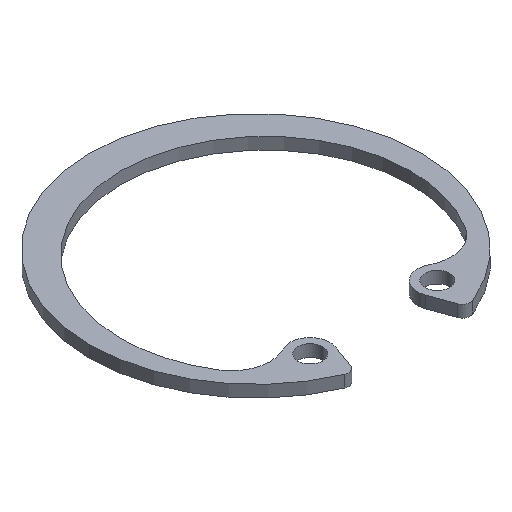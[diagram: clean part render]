
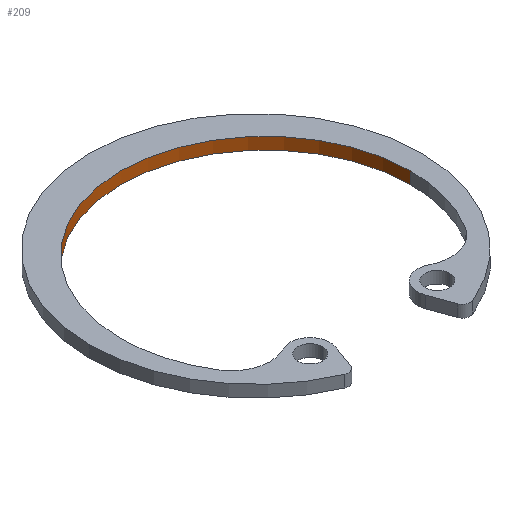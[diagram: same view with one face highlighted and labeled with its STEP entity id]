
A CAD part, isometric view. The second image highlights one B-rep face of the part: STEP entity #209.
In plain terms, the highlighted cylindrical face has radius 14.6 mm (diameter 29.199 mm), a partial arc.
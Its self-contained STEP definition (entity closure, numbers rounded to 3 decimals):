
#15 = CIRCLE ( 'NONE', #135, 14.6 ) ;
#21 = CARTESIAN_POINT ( 'NONE',  ( 14.6, -1., -0.6 ) ) ;
#37 = EDGE_CURVE ( 'NONE', #615, #424, #297, .T. ) ;
#42 = AXIS2_PLACEMENT_3D ( 'NONE', #620, #249, #412 ) ;
#67 = CARTESIAN_POINT ( 'NONE',  ( -14.6, -1., -0.6 ) ) ;
#68 = CARTESIAN_POINT ( 'NONE',  ( -14.6, -1., -0.6 ) ) ;
#122 = LINE ( 'NONE', #67, #317 ) ;
#135 = AXIS2_PLACEMENT_3D ( 'NONE', #693, #192, #524 ) ;
#144 = EDGE_LOOP ( 'NONE', ( #557, #586, #534, #206 ) ) ;
#192 = DIRECTION ( 'NONE',  ( 0., 0., -1. ) ) ;
#200 = CIRCLE ( 'NONE', #42, 14.6 ) ;
#205 = CARTESIAN_POINT ( 'NONE',  ( -14.6, -1., 0.6 ) ) ;
#206 = ORIENTED_EDGE ( 'NONE', *, *, #647, .F. ) ;
#209 = ADVANCED_FACE ( 'NONE', ( #641 ), #532, .F. ) ;
#249 = DIRECTION ( 'NONE',  ( 0., 0., -1. ) ) ;
#252 = DIRECTION ( 'NONE',  ( 0., 0., 1. ) ) ;
#278 = EDGE_CURVE ( 'NONE', #329, #615, #15, .T. ) ;
#291 = DIRECTION ( 'NONE',  ( 1., 0., 0. ) ) ;
#297 = LINE ( 'NONE', #567, #427 ) ;
#317 = VECTOR ( 'NONE', #472, 1000. ) ;
#329 = VERTEX_POINT ( 'NONE', #68 ) ;
#412 = DIRECTION ( 'NONE',  ( -1., 0., 0. ) ) ;
#424 = VERTEX_POINT ( 'NONE', #488 ) ;
#427 = VECTOR ( 'NONE', #252, 1000. ) ;
#461 = CARTESIAN_POINT ( 'NONE',  ( 0., -1., -0.6 ) ) ;
#469 = DIRECTION ( 'NONE',  ( 0., 0., 1. ) ) ;
#472 = DIRECTION ( 'NONE',  ( 0., 0., 1. ) ) ;
#484 = VERTEX_POINT ( 'NONE', #205 ) ;
#488 = CARTESIAN_POINT ( 'NONE',  ( 14.6, -1., 0.6 ) ) ;
#524 = DIRECTION ( 'NONE',  ( -1., 0., 0. ) ) ;
#532 = CYLINDRICAL_SURFACE ( 'NONE', #678, 14.6 ) ;
#534 = ORIENTED_EDGE ( 'NONE', *, *, #37, .T. ) ;
#557 = ORIENTED_EDGE ( 'NONE', *, *, #696, .F. ) ;
#567 = CARTESIAN_POINT ( 'NONE',  ( 14.6, -1., -0.6 ) ) ;
#586 = ORIENTED_EDGE ( 'NONE', *, *, #278, .T. ) ;
#615 = VERTEX_POINT ( 'NONE', #21 ) ;
#620 = CARTESIAN_POINT ( 'NONE',  ( 0., -1., 0.6 ) ) ;
#641 = FACE_OUTER_BOUND ( 'NONE', #144, .T. ) ;
#647 = EDGE_CURVE ( 'NONE', #484, #424, #200, .T. ) ;
#678 = AXIS2_PLACEMENT_3D ( 'NONE', #461, #469, #291 ) ;
#693 = CARTESIAN_POINT ( 'NONE',  ( 0., -1., -0.6 ) ) ;
#696 = EDGE_CURVE ( 'NONE', #329, #484, #122, .T. ) ;
